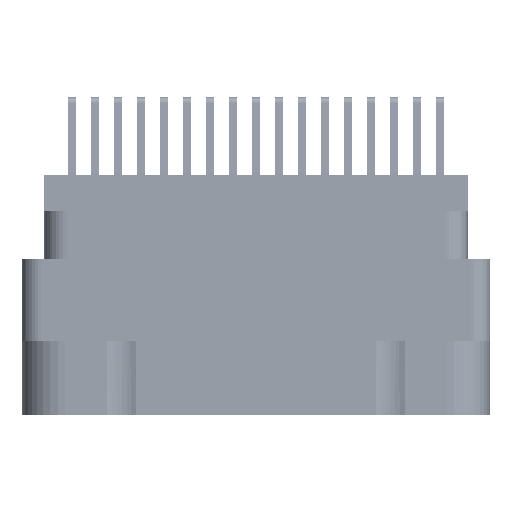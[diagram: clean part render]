
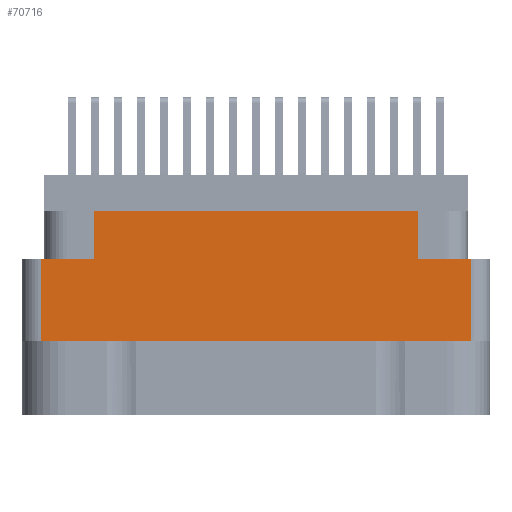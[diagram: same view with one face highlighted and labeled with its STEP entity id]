
A CAD part, left-side view. The second image highlights one B-rep face of the part: STEP entity #70716.
In plain terms, the highlighted planar face has unit normal (-1, 0, 0).
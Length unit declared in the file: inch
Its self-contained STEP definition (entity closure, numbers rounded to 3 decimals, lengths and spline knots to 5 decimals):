
#1574 = CARTESIAN_POINT ( 'NONE',  ( -1.375, 0., -0.274 ) ) ;
#3184 = VECTOR ( 'NONE', #84464, 39.37008 ) ;
#4812 = CARTESIAN_POINT ( 'NONE',  ( -1.375, 0.5285, -0.274 ) ) ;
#6029 = VERTEX_POINT ( 'NONE', #55042 ) ;
#7658 = ORIENTED_EDGE ( 'NONE', *, *, #60541, .T. ) ;
#8250 = VECTOR ( 'NONE', #67251, 39.37008 ) ;
#8738 = ORIENTED_EDGE ( 'NONE', *, *, #37124, .F. ) ;
#9274 = DIRECTION ( 'NONE',  ( 0., 0., 1. ) ) ;
#10187 = EDGE_LOOP ( 'NONE', ( #58042, #20567, #7658, #19064, #34860, #66173, #8738, #13385 ) ) ;
#11316 = DIRECTION ( 'NONE',  ( 0., 0., 1. ) ) ;
#12427 = EDGE_CURVE ( 'NONE', #21574, #48495, #21208, .T. ) ;
#12498 = CARTESIAN_POINT ( 'NONE',  ( -1.375, -0.7005, -0.54 ) ) ;
#12753 = DIRECTION ( 'NONE',  ( 0., 0., -1. ) ) ;
#12951 = CARTESIAN_POINT ( 'NONE',  ( -1.375, 0., -0.54 ) ) ;
#13385 = ORIENTED_EDGE ( 'NONE', *, *, #58274, .F. ) ;
#14590 = CARTESIAN_POINT ( 'NONE',  ( -1.375, 0.7005, -0.274 ) ) ;
#14633 = VECTOR ( 'NONE', #84028, 39.37008 ) ;
#14888 = VECTOR ( 'NONE', #11316, 39.37008 ) ;
#15500 = VECTOR ( 'NONE', #40983, 39.37008 ) ;
#19064 = ORIENTED_EDGE ( 'NONE', *, *, #84158, .T. ) ;
#19963 = VERTEX_POINT ( 'NONE', #40161 ) ;
#20567 = ORIENTED_EDGE ( 'NONE', *, *, #12427, .T. ) ;
#21208 = LINE ( 'NONE', #25917, #55941 ) ;
#21574 = VERTEX_POINT ( 'NONE', #14590 ) ;
#22351 = LINE ( 'NONE', #36033, #64428 ) ;
#22353 = CARTESIAN_POINT ( 'NONE',  ( -1.375, 0.5285, -0.117 ) ) ;
#22715 = CARTESIAN_POINT ( 'NONE',  ( -1.375, -0.5285, -0.117 ) ) ;
#24036 = EDGE_CURVE ( 'NONE', #21574, #19963, #52398, .T. ) ;
#25917 = CARTESIAN_POINT ( 'NONE',  ( -1.375, 0.7005, -0.78 ) ) ;
#27125 = VERTEX_POINT ( 'NONE', #41631 ) ;
#27366 = LINE ( 'NONE', #64130, #3184 ) ;
#30198 = CARTESIAN_POINT ( 'NONE',  ( -1.375, 0.7625, -0.117 ) ) ;
#31374 = DIRECTION ( 'NONE',  ( 0., 0., 1. ) ) ;
#34752 = CARTESIAN_POINT ( 'NONE',  ( -1.375, 0.7005, -0.54 ) ) ;
#34860 = ORIENTED_EDGE ( 'NONE', *, *, #79544, .F. ) ;
#35207 = LINE ( 'NONE', #12951, #8250 ) ;
#36033 = CARTESIAN_POINT ( 'NONE',  ( -1.375, -0.5285, -0.274 ) ) ;
#37124 = EDGE_CURVE ( 'NONE', #70538, #77623, #48294, .T. ) ;
#40161 = CARTESIAN_POINT ( 'NONE',  ( -1.375, 0.5285, -0.274 ) ) ;
#40715 = AXIS2_PLACEMENT_3D ( 'NONE', #44439, #43860, #31374 ) ;
#40983 = DIRECTION ( 'NONE',  ( 0., -1., 0. ) ) ;
#41631 = CARTESIAN_POINT ( 'NONE',  ( -1.375, -0.5285, -0.274 ) ) ;
#43860 = DIRECTION ( 'NONE',  ( -1., 0., 0. ) ) ;
#44439 = CARTESIAN_POINT ( 'NONE',  ( -1.375, -0.7625, -0.78 ) ) ;
#47876 = VERTEX_POINT ( 'NONE', #12498 ) ;
#48294 = LINE ( 'NONE', #30198, #14633 ) ;
#48495 = VERTEX_POINT ( 'NONE', #34752 ) ;
#48837 = LINE ( 'NONE', #62345, #56167 ) ;
#52398 = LINE ( 'NONE', #1574, #15500 ) ;
#55042 = CARTESIAN_POINT ( 'NONE',  ( -1.375, -0.7005, -0.274 ) ) ;
#55941 = VECTOR ( 'NONE', #12753, 39.37008 ) ;
#56167 = VECTOR ( 'NONE', #56503, 39.37008 ) ;
#56503 = DIRECTION ( 'NONE',  ( 0., 0., 1. ) ) ;
#58042 = ORIENTED_EDGE ( 'NONE', *, *, #24036, .F. ) ;
#58274 = EDGE_CURVE ( 'NONE', #19963, #70538, #59098, .T. ) ;
#59098 = LINE ( 'NONE', #4812, #14888 ) ;
#60541 = EDGE_CURVE ( 'NONE', #48495, #47876, #35207, .T. ) ;
#62345 = CARTESIAN_POINT ( 'NONE',  ( -1.375, -0.7005, -0.78 ) ) ;
#64130 = CARTESIAN_POINT ( 'NONE',  ( -1.375, 0., -0.274 ) ) ;
#64428 = VECTOR ( 'NONE', #9274, 39.37008 ) ;
#66173 = ORIENTED_EDGE ( 'NONE', *, *, #85133, .T. ) ;
#67173 = FACE_OUTER_BOUND ( 'NONE', #10187, .T. ) ;
#67251 = DIRECTION ( 'NONE',  ( 0., -1., 0. ) ) ;
#70538 = VERTEX_POINT ( 'NONE', #22353 ) ;
#70716 = ADVANCED_FACE ( 'NONE', ( #67173 ), #84637, .T. ) ;
#77623 = VERTEX_POINT ( 'NONE', #22715 ) ;
#79544 = EDGE_CURVE ( 'NONE', #27125, #6029, #27366, .T. ) ;
#84028 = DIRECTION ( 'NONE',  ( 0., -1., 0. ) ) ;
#84158 = EDGE_CURVE ( 'NONE', #47876, #6029, #48837, .T. ) ;
#84464 = DIRECTION ( 'NONE',  ( 0., -1., 0. ) ) ;
#84637 = PLANE ( 'NONE',  #40715 ) ;
#85133 = EDGE_CURVE ( 'NONE', #27125, #77623, #22351, .T. ) ;
